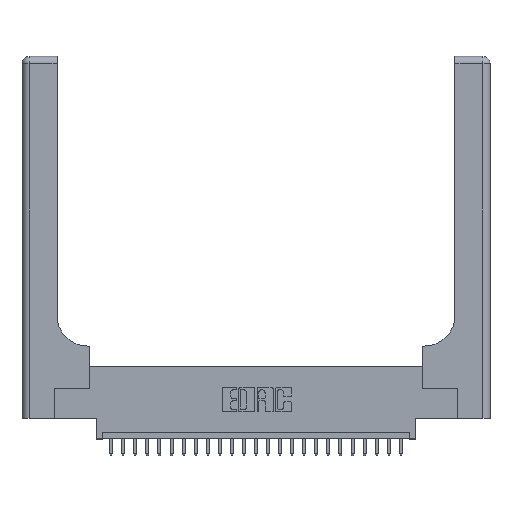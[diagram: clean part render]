
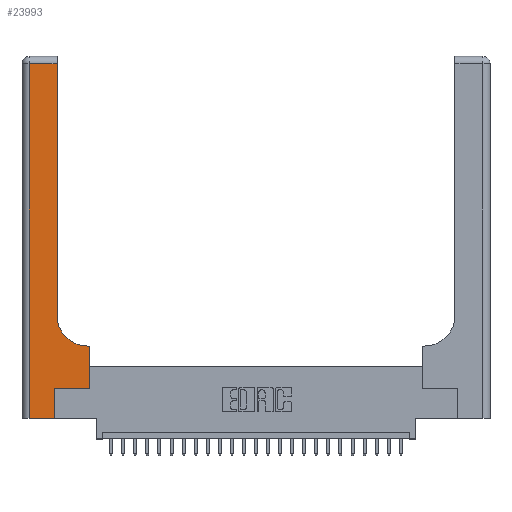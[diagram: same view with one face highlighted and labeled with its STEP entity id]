
A CAD part, top view. The second image highlights one B-rep face of the part: STEP entity #23993.
In plain terms, the highlighted planar face has unit normal (0, 0, 1).
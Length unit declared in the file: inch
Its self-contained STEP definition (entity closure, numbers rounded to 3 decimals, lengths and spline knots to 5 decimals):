
#402 = ORIENTED_EDGE ( 'NONE', *, *, #13785, .T. ) ;
#407 = ORIENTED_EDGE ( 'NONE', *, *, #24525, .T. ) ;
#782 = DIRECTION ( 'NONE',  ( 0., -1., 0. ) ) ;
#927 = VECTOR ( 'NONE', #4435, 39.37008 ) ;
#938 = EDGE_CURVE ( 'NONE', #22442, #20825, #20755, .T. ) ;
#1028 = EDGE_LOOP ( 'NONE', ( #1845, #13768, #402, #13964, #26139, #20647, #24971, #407, #13846 ) ) ;
#1845 = ORIENTED_EDGE ( 'NONE', *, *, #19043, .T. ) ;
#2024 = CARTESIAN_POINT ( 'NONE',  ( 0.269, 0.25, 0.37 ) ) ;
#2053 = EDGE_CURVE ( 'NONE', #13282, #12469, #4932, .T. ) ;
#2261 = DIRECTION ( 'NONE',  ( 1., 0., 0. ) ) ;
#2410 = CARTESIAN_POINT ( 'NONE',  ( 0.269, 0., 0.37 ) ) ;
#4296 = CARTESIAN_POINT ( 'NONE',  ( 0., 0., 0.37 ) ) ;
#4315 = DIRECTION ( 'NONE',  ( 1., 0., 0. ) ) ;
#4435 = DIRECTION ( 'NONE',  ( 0., 1., 0. ) ) ;
#4461 = VERTEX_POINT ( 'NONE', #6974 ) ;
#4781 = AXIS2_PLACEMENT_3D ( 'NONE', #26121, #15737, #13771 ) ;
#4929 = LINE ( 'NONE', #16928, #25993 ) ;
#4932 = LINE ( 'NONE', #25844, #9062 ) ;
#5250 = DIRECTION ( 'NONE',  ( 0., 0., -1. ) ) ;
#5557 = CARTESIAN_POINT ( 'NONE',  ( 0.5585, 0.25, 0.37 ) ) ;
#6419 = VERTEX_POINT ( 'NONE', #17689 ) ;
#6974 = CARTESIAN_POINT ( 'NONE',  ( 0.5415, 0.6, 0.37 ) ) ;
#7136 = EDGE_CURVE ( 'NONE', #12469, #22442, #8826, .T. ) ;
#8377 = CARTESIAN_POINT ( 'NONE',  ( 0.06, 3., 0.37 ) ) ;
#8413 = CARTESIAN_POINT ( 'NONE',  ( 0.5585, 0.6, 0.37 ) ) ;
#8628 = VECTOR ( 'NONE', #26248, 39.37008 ) ;
#8826 = LINE ( 'NONE', #2024, #17108 ) ;
#8929 = EDGE_CURVE ( 'NONE', #21144, #6419, #4929, .T. ) ;
#9062 = VECTOR ( 'NONE', #23066, 39.37008 ) ;
#9340 = CARTESIAN_POINT ( 'NONE',  ( 0.5415, 0.85, 0.37 ) ) ;
#9789 = LINE ( 'NONE', #8377, #21586 ) ;
#9902 = LINE ( 'NONE', #15263, #13093 ) ;
#10873 = DIRECTION ( 'NONE',  ( -1., 0., 0. ) ) ;
#12469 = VERTEX_POINT ( 'NONE', #20275 ) ;
#13093 = VECTOR ( 'NONE', #17333, 39.37008 ) ;
#13282 = VERTEX_POINT ( 'NONE', #2410 ) ;
#13583 = PLANE ( 'NONE',  #4781 ) ;
#13768 = ORIENTED_EDGE ( 'NONE', *, *, #8929, .T. ) ;
#13771 = DIRECTION ( 'NONE',  ( -1., 0., 0. ) ) ;
#13785 = EDGE_CURVE ( 'NONE', #6419, #17765, #9789, .T. ) ;
#13846 = ORIENTED_EDGE ( 'NONE', *, *, #21637, .T. ) ;
#13964 = ORIENTED_EDGE ( 'NONE', *, *, #14476, .T. ) ;
#14028 = CARTESIAN_POINT ( 'NONE',  ( 0.06, 0., 0.37 ) ) ;
#14382 = FACE_OUTER_BOUND ( 'NONE', #1028, .T. ) ;
#14399 = CARTESIAN_POINT ( 'NONE',  ( 0.2915, 3., 0.37 ) ) ;
#14476 = EDGE_CURVE ( 'NONE', #17765, #13282, #22821, .T. ) ;
#14837 = CIRCLE ( 'NONE', #15284, 0.25 ) ;
#15150 = CARTESIAN_POINT ( 'NONE',  ( 0.2915, 0.85, 0.37 ) ) ;
#15263 = CARTESIAN_POINT ( 'NONE',  ( 0.2915, 0.6, 0.37 ) ) ;
#15284 = AXIS2_PLACEMENT_3D ( 'NONE', #9340, #5250, #25684 ) ;
#15737 = DIRECTION ( 'NONE',  ( 0., 0., -1. ) ) ;
#16340 = VERTEX_POINT ( 'NONE', #15150 ) ;
#16928 = CARTESIAN_POINT ( 'NONE',  ( 0., 2.94, 0.37 ) ) ;
#17108 = VECTOR ( 'NONE', #4315, 39.37008 ) ;
#17333 = DIRECTION ( 'NONE',  ( -1., 0., 0. ) ) ;
#17689 = CARTESIAN_POINT ( 'NONE',  ( 0.06, 2.94, 0.37 ) ) ;
#17765 = VERTEX_POINT ( 'NONE', #14028 ) ;
#18689 = VECTOR ( 'NONE', #2261, 39.37008 ) ;
#19043 = EDGE_CURVE ( 'NONE', #16340, #21144, #19420, .T. ) ;
#19420 = LINE ( 'NONE', #14399, #927 ) ;
#19976 = CARTESIAN_POINT ( 'NONE',  ( 0.2915, 2.94, 0.37 ) ) ;
#20275 = CARTESIAN_POINT ( 'NONE',  ( 0.269, 0.25, 0.37 ) ) ;
#20647 = ORIENTED_EDGE ( 'NONE', *, *, #7136, .T. ) ;
#20663 = CARTESIAN_POINT ( 'NONE',  ( 0.5585, 0.25, 0.37 ) ) ;
#20755 = LINE ( 'NONE', #20663, #8628 ) ;
#20825 = VERTEX_POINT ( 'NONE', #8413 ) ;
#21144 = VERTEX_POINT ( 'NONE', #19976 ) ;
#21586 = VECTOR ( 'NONE', #782, 39.37008 ) ;
#21637 = EDGE_CURVE ( 'NONE', #4461, #16340, #14837, .T. ) ;
#22442 = VERTEX_POINT ( 'NONE', #5557 ) ;
#22821 = LINE ( 'NONE', #4296, #18689 ) ;
#23066 = DIRECTION ( 'NONE',  ( 0., 1., 0. ) ) ;
#23993 = ADVANCED_FACE ( 'NONE', ( #14382 ), #13583, .F. ) ;
#24525 = EDGE_CURVE ( 'NONE', #20825, #4461, #9902, .T. ) ;
#24971 = ORIENTED_EDGE ( 'NONE', *, *, #938, .T. ) ;
#25684 = DIRECTION ( 'NONE',  ( 1., 0., 0. ) ) ;
#25844 = CARTESIAN_POINT ( 'NONE',  ( 0.269, 0., 0.37 ) ) ;
#25993 = VECTOR ( 'NONE', #10873, 39.37008 ) ;
#26121 = CARTESIAN_POINT ( 'NONE',  ( 0., 3., 0.37 ) ) ;
#26139 = ORIENTED_EDGE ( 'NONE', *, *, #2053, .T. ) ;
#26248 = DIRECTION ( 'NONE',  ( 0., 1., 0. ) ) ;
